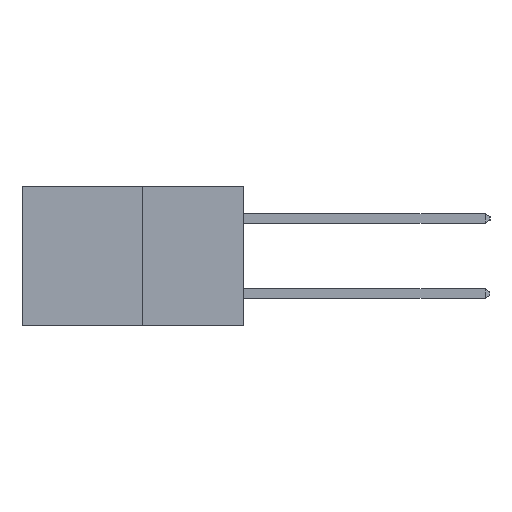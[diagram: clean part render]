
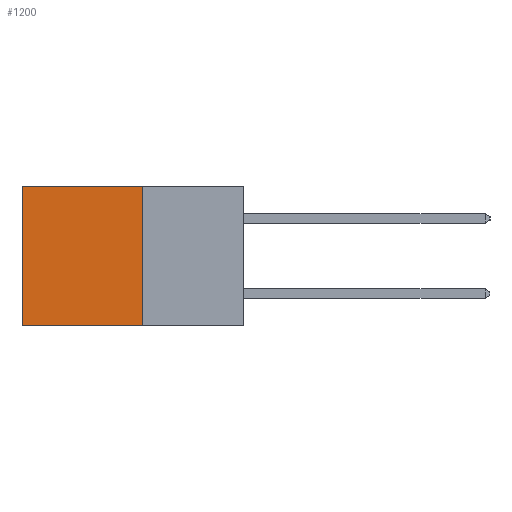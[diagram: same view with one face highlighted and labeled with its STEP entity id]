
A CAD part, left-side view. The second image highlights one B-rep face of the part: STEP entity #1200.
In plain terms, the highlighted planar face has unit normal (-1, 0, 0).
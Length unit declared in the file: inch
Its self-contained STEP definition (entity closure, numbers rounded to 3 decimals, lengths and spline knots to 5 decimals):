
#195 = VERTEX_POINT ( 'NONE', #17898 ) ;
#469 = DIRECTION ( 'NONE',  ( 0., 1., 0. ) ) ;
#1134 = CARTESIAN_POINT ( 'NONE',  ( 0.277, 0.27, -0.37 ) ) ;
#1200 = ADVANCED_FACE ( 'NONE', ( #5537 ), #13740, .F. ) ;
#1619 = CARTESIAN_POINT ( 'NONE',  ( 0.277, 0.27, 0. ) ) ;
#3590 = LINE ( 'NONE', #1619, #7893 ) ;
#5159 = EDGE_CURVE ( 'NONE', #5286, #7876, #3590, .T. ) ;
#5286 = VERTEX_POINT ( 'NONE', #10635 ) ;
#5537 = FACE_OUTER_BOUND ( 'NONE', #13777, .T. ) ;
#6042 = VECTOR ( 'NONE', #9079, 39.37008 ) ;
#6057 = VECTOR ( 'NONE', #19197, 39.37008 ) ;
#6779 = DIRECTION ( 'NONE',  ( 0., 0., -1. ) ) ;
#7694 = VECTOR ( 'NONE', #13554, 39.37008 ) ;
#7876 = VERTEX_POINT ( 'NONE', #9933 ) ;
#7893 = VECTOR ( 'NONE', #469, 39.37008 ) ;
#8547 = ORIENTED_EDGE ( 'NONE', *, *, #8830, .T. ) ;
#8830 = EDGE_CURVE ( 'NONE', #7876, #195, #16079, .T. ) ;
#9079 = DIRECTION ( 'NONE',  ( 0., 0., -1. ) ) ;
#9117 = ORIENTED_EDGE ( 'NONE', *, *, #15803, .F. ) ;
#9465 = CARTESIAN_POINT ( 'NONE',  ( 0.277, 0.59, -0.37 ) ) ;
#9933 = CARTESIAN_POINT ( 'NONE',  ( 0.277, 0.59, 0. ) ) ;
#10006 = AXIS2_PLACEMENT_3D ( 'NONE', #15363, #17823, #6779 ) ;
#10171 = EDGE_CURVE ( 'NONE', #19083, #195, #11377, .T. ) ;
#10635 = CARTESIAN_POINT ( 'NONE',  ( 0.277, 0.27, 0. ) ) ;
#11377 = LINE ( 'NONE', #13630, #7694 ) ;
#11455 = LINE ( 'NONE', #17530, #6057 ) ;
#13301 = ORIENTED_EDGE ( 'NONE', *, *, #10171, .F. ) ;
#13554 = DIRECTION ( 'NONE',  ( 0., 1., 0. ) ) ;
#13630 = CARTESIAN_POINT ( 'NONE',  ( 0.277, 0.27, -0.37 ) ) ;
#13740 = PLANE ( 'NONE',  #10006 ) ;
#13777 = EDGE_LOOP ( 'NONE', ( #8547, #13301, #9117, #13858 ) ) ;
#13858 = ORIENTED_EDGE ( 'NONE', *, *, #5159, .T. ) ;
#15363 = CARTESIAN_POINT ( 'NONE',  ( 0.277, 0.27, -0.37 ) ) ;
#15803 = EDGE_CURVE ( 'NONE', #5286, #19083, #11455, .T. ) ;
#16079 = LINE ( 'NONE', #9465, #6042 ) ;
#17530 = CARTESIAN_POINT ( 'NONE',  ( 0.277, 0.27, -0.37 ) ) ;
#17823 = DIRECTION ( 'NONE',  ( 1., 0., 0. ) ) ;
#17898 = CARTESIAN_POINT ( 'NONE',  ( 0.277, 0.59, -0.37 ) ) ;
#19083 = VERTEX_POINT ( 'NONE', #1134 ) ;
#19197 = DIRECTION ( 'NONE',  ( 0., 0., -1. ) ) ;
